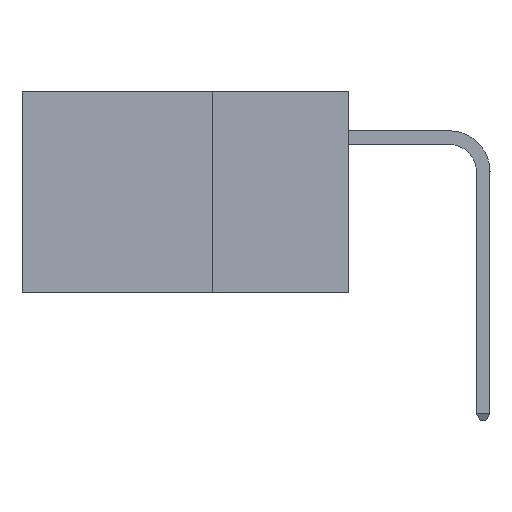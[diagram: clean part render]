
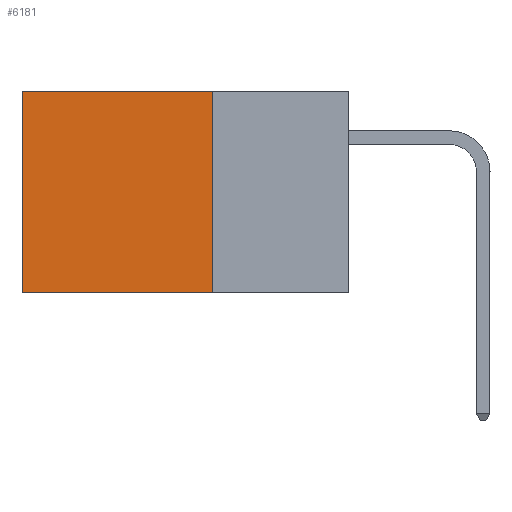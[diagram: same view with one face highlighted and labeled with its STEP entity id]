
A CAD part, left-side view. The second image highlights one B-rep face of the part: STEP entity #6181.
In plain terms, the highlighted planar face has unit normal (-1, 0, 0).
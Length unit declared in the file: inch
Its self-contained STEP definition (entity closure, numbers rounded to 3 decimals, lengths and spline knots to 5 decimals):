
#1276 = CARTESIAN_POINT ( 'NONE',  ( 0.2875, 0.6, 0. ) ) ;
#4126 = EDGE_CURVE ( 'NONE', #26058, #13230, #23416, .T. ) ;
#4265 = DIRECTION ( 'NONE',  ( 1., 0., 0. ) ) ;
#5598 = DIRECTION ( 'NONE',  ( 0., 0., -1. ) ) ;
#6181 = ADVANCED_FACE ( 'NONE', ( #43622 ), #32454, .F. ) ;
#6552 = EDGE_CURVE ( 'NONE', #38567, #30181, #29155, .T. ) ;
#7165 = DIRECTION ( 'NONE',  ( 0., 0., -1. ) ) ;
#10180 = CARTESIAN_POINT ( 'NONE',  ( 0.2875, 0.6, 0. ) ) ;
#10373 = CARTESIAN_POINT ( 'NONE',  ( 0.2875, 0.25, 0. ) ) ;
#11164 = ORIENTED_EDGE ( 'NONE', *, *, #32492, .F. ) ;
#11990 = DIRECTION ( 'NONE',  ( 0., 1., 0. ) ) ;
#13230 = VERTEX_POINT ( 'NONE', #22413 ) ;
#15918 = DIRECTION ( 'NONE',  ( 0., 0., -1. ) ) ;
#16195 = VECTOR ( 'NONE', #11990, 39.37008 ) ;
#16593 = LINE ( 'NONE', #10373, #43714 ) ;
#19777 = VECTOR ( 'NONE', #7165, 39.37008 ) ;
#20608 = LINE ( 'NONE', #26095, #16195 ) ;
#22413 = CARTESIAN_POINT ( 'NONE',  ( 0.2875, 0.6, -0.37 ) ) ;
#23416 = LINE ( 'NONE', #1276, #35049 ) ;
#25343 = CARTESIAN_POINT ( 'NONE',  ( 0.2875, 0.25, 0. ) ) ;
#26058 = VERTEX_POINT ( 'NONE', #10180 ) ;
#26095 = CARTESIAN_POINT ( 'NONE',  ( 0.2875, 0.25, -0.37 ) ) ;
#26266 = ORIENTED_EDGE ( 'NONE', *, *, #28488, .T. ) ;
#27484 = ORIENTED_EDGE ( 'NONE', *, *, #4126, .T. ) ;
#27755 = EDGE_LOOP ( 'NONE', ( #27484, #11164, #32369, #26266 ) ) ;
#28488 = EDGE_CURVE ( 'NONE', #38567, #26058, #16593, .T. ) ;
#29155 = LINE ( 'NONE', #45720, #19777 ) ;
#30181 = VERTEX_POINT ( 'NONE', #43713 ) ;
#32033 = DIRECTION ( 'NONE',  ( 0., 1., 0. ) ) ;
#32369 = ORIENTED_EDGE ( 'NONE', *, *, #6552, .F. ) ;
#32454 = PLANE ( 'NONE',  #36837 ) ;
#32492 = EDGE_CURVE ( 'NONE', #30181, #13230, #20608, .T. ) ;
#35049 = VECTOR ( 'NONE', #5598, 39.37008 ) ;
#36837 = AXIS2_PLACEMENT_3D ( 'NONE', #25343, #4265, #15918 ) ;
#38567 = VERTEX_POINT ( 'NONE', #39657 ) ;
#39657 = CARTESIAN_POINT ( 'NONE',  ( 0.2875, 0.25, 0. ) ) ;
#43622 = FACE_OUTER_BOUND ( 'NONE', #27755, .T. ) ;
#43713 = CARTESIAN_POINT ( 'NONE',  ( 0.2875, 0.25, -0.37 ) ) ;
#43714 = VECTOR ( 'NONE', #32033, 39.37008 ) ;
#45720 = CARTESIAN_POINT ( 'NONE',  ( 0.2875, 0.25, 0. ) ) ;
